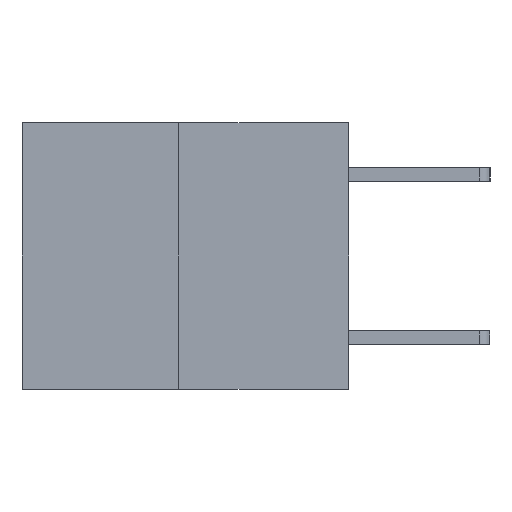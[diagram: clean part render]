
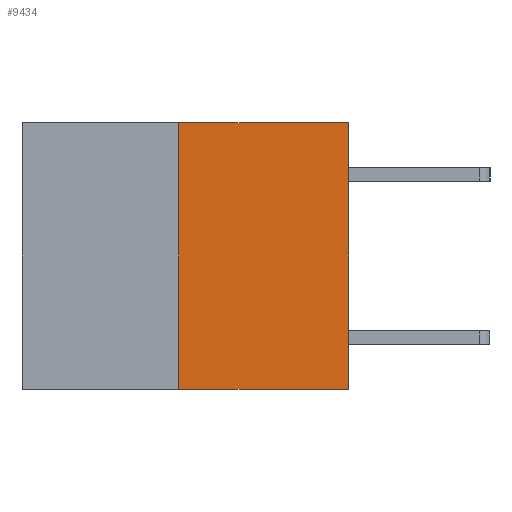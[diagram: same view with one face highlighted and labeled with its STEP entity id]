
A CAD part, left-side view. The second image highlights one B-rep face of the part: STEP entity #9434.
In plain terms, the highlighted planar face has unit normal (-1, 0, 0).
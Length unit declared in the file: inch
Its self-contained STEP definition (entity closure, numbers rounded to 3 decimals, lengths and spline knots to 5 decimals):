
#227 = DIRECTION ( 'NONE',  ( 0., -1., 0. ) ) ;
#346 = CARTESIAN_POINT ( 'NONE',  ( 0., 0.6, 0. ) ) ;
#934 = VECTOR ( 'NONE', #227, 39.37008 ) ;
#1064 = PLANE ( 'NONE',  #2444 ) ;
#1181 = EDGE_CURVE ( 'NONE', #9000, #5400, #5894, .T. ) ;
#1317 = EDGE_CURVE ( 'NONE', #5400, #9011, #5172, .T. ) ;
#1549 = EDGE_LOOP ( 'NONE', ( #2795, #2820, #3075, #8376 ) ) ;
#1596 = VERTEX_POINT ( 'NONE', #5329 ) ;
#1997 = LINE ( 'NONE', #2231, #8257 ) ;
#2231 = CARTESIAN_POINT ( 'NONE',  ( 0., 0.6, 0. ) ) ;
#2236 = VECTOR ( 'NONE', #4910, 39.37008 ) ;
#2444 = AXIS2_PLACEMENT_3D ( 'NONE', #346, #8525, #6346 ) ;
#2631 = CARTESIAN_POINT ( 'NONE',  ( 0., 0., -0.49 ) ) ;
#2795 = ORIENTED_EDGE ( 'NONE', *, *, #6595, .F. ) ;
#2820 = ORIENTED_EDGE ( 'NONE', *, *, #1181, .T. ) ;
#2852 = DIRECTION ( 'NONE',  ( 0., -1., 0. ) ) ;
#3075 = ORIENTED_EDGE ( 'NONE', *, *, #1317, .T. ) ;
#3652 = CARTESIAN_POINT ( 'NONE',  ( 0., 0.312, -0.49 ) ) ;
#4910 = DIRECTION ( 'NONE',  ( 0., 0., 1. ) ) ;
#5135 = FACE_OUTER_BOUND ( 'NONE', #1549, .T. ) ;
#5172 = LINE ( 'NONE', #8596, #2236 ) ;
#5329 = CARTESIAN_POINT ( 'NONE',  ( 0., 0.312, 0. ) ) ;
#5400 = VERTEX_POINT ( 'NONE', #2631 ) ;
#5894 = LINE ( 'NONE', #6288, #934 ) ;
#6169 = DIRECTION ( 'NONE',  ( 0., 0., 1. ) ) ;
#6288 = CARTESIAN_POINT ( 'NONE',  ( 0., 0.6, -0.49 ) ) ;
#6333 = VECTOR ( 'NONE', #6169, 39.37008 ) ;
#6346 = DIRECTION ( 'NONE',  ( 0., 0., -1. ) ) ;
#6595 = EDGE_CURVE ( 'NONE', #9000, #1596, #8737, .T. ) ;
#8257 = VECTOR ( 'NONE', #2852, 39.37008 ) ;
#8376 = ORIENTED_EDGE ( 'NONE', *, *, #8857, .F. ) ;
#8525 = DIRECTION ( 'NONE',  ( 1., 0., 0. ) ) ;
#8596 = CARTESIAN_POINT ( 'NONE',  ( 0., 0., 0. ) ) ;
#8737 = LINE ( 'NONE', #9240, #6333 ) ;
#8857 = EDGE_CURVE ( 'NONE', #1596, #9011, #1997, .T. ) ;
#8948 = CARTESIAN_POINT ( 'NONE',  ( 0., 0., 0. ) ) ;
#9000 = VERTEX_POINT ( 'NONE', #3652 ) ;
#9011 = VERTEX_POINT ( 'NONE', #8948 ) ;
#9240 = CARTESIAN_POINT ( 'NONE',  ( 0., 0.312, -0.49 ) ) ;
#9434 = ADVANCED_FACE ( 'NONE', ( #5135 ), #1064, .F. ) ;
